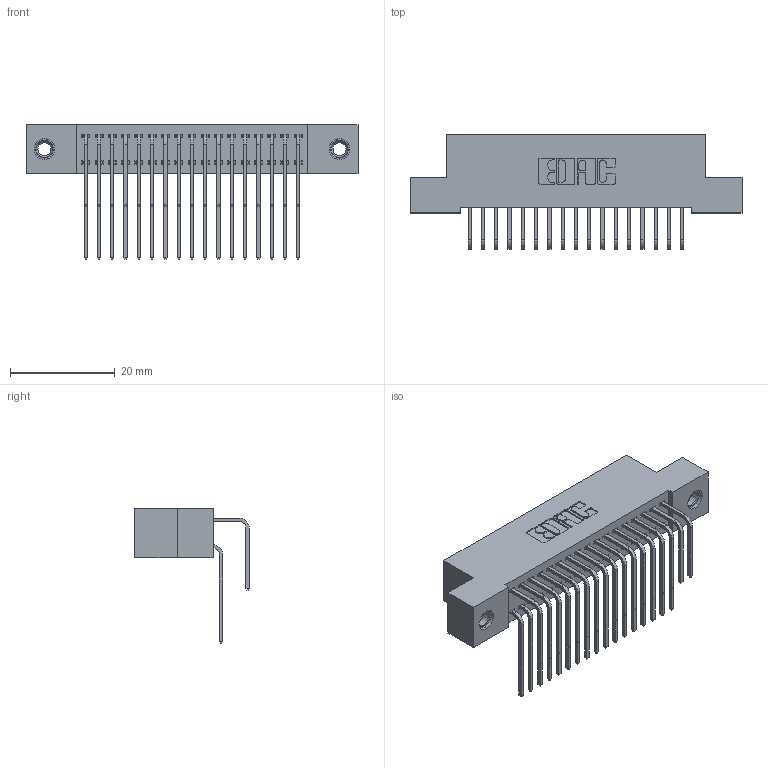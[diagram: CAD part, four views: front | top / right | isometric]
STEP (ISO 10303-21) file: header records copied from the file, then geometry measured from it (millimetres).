
FILE_DESCRIPTION (( 'STEP AP203' ), '1' );
FILE_NAME ('342-034-558-207.STEP', '2018-08-11T19:01:48', ( '' ), ( '' ), 'SwSTEP 2.0', 'SolidWorks 2016', '' );
FILE_SCHEMA (( 'CONFIG_CONTROL_DESIGN' ));
Length unit declared in the file: inch
Products named in the file (5): 345-292-001_558 559 Tail - 1; 345-292-001_558 Tail - 2; 345-250-001_345-250-005-103; 342-034-558-207; 342 Part_TI
Assembly tree (37 placements, depth 2):
  342-034-558-207
    342 Part_TI
    345-292-001_558 559 Tail - 1  x17
    345-292-001_558 Tail - 2  x17
    345-250-001_345-250-005-103  x2
Bounding box: 63.5 x 21.91 x 25.78 mm (x, y, z)
Volume: 5770.6 mm3; surface area: 9690.1 mm2
Topology: 37 solids, 37 shells, 2006 faces, 5909 edges, 3886 vertices
Faces by surface type: plane 1390, cylinder 600, cone 12, torus 4
Entity records: 17008 total; most frequent: CARTESIAN_POINT 2880, ORIENTED_EDGE 2758, DIRECTION 2517, EDGE_CURVE 1379, LINE 1191, VECTOR 1191, VERTEX_POINT 912, AXIS2_PLACEMENT_3D 663
